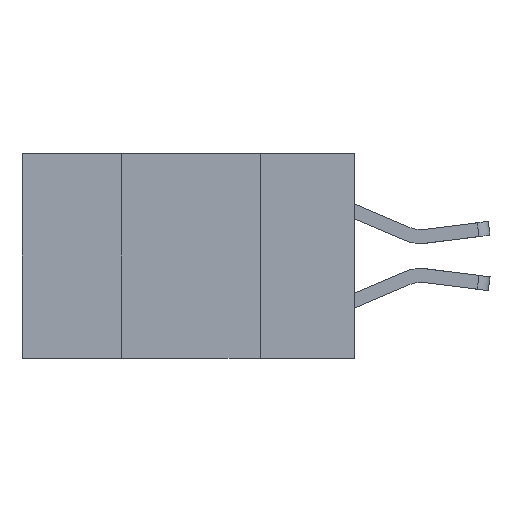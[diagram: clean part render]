
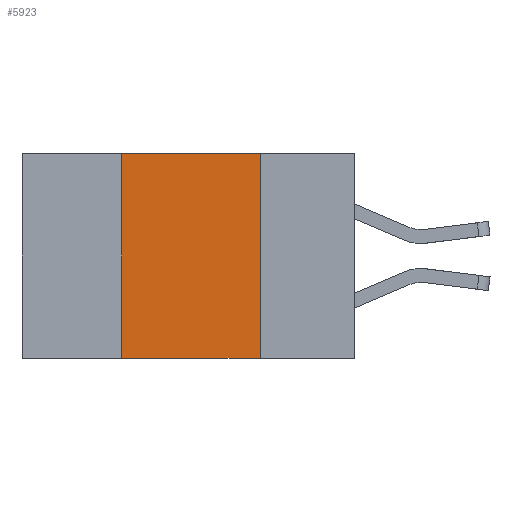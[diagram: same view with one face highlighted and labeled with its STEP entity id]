
A CAD part, left-side view. The second image highlights one B-rep face of the part: STEP entity #5923.
In plain terms, the highlighted planar face has unit normal (-1, 0, 0).
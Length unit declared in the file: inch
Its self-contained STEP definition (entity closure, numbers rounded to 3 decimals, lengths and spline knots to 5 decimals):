
#590 = CARTESIAN_POINT ( 'NONE',  ( 0., 0.17, 0. ) ) ;
#648 = VERTEX_POINT ( 'NONE', #7465 ) ;
#1519 = CARTESIAN_POINT ( 'NONE',  ( 0., 0.42, 0. ) ) ;
#1702 = EDGE_CURVE ( 'NONE', #5550, #648, #6798, .T. ) ;
#1976 = VECTOR ( 'NONE', #5303, 39.37008 ) ;
#2070 = EDGE_CURVE ( 'NONE', #648, #4972, #3769, .T. ) ;
#2094 = CARTESIAN_POINT ( 'NONE',  ( 0., 0.17, -0.37 ) ) ;
#2158 = CARTESIAN_POINT ( 'NONE',  ( 0., 0.6, -0.37 ) ) ;
#2169 = EDGE_CURVE ( 'NONE', #8180, #4972, #6313, .T. ) ;
#2476 = ORIENTED_EDGE ( 'NONE', *, *, #2169, .T. ) ;
#2839 = EDGE_LOOP ( 'NONE', ( #8367, #7723, #8049, #2476 ) ) ;
#3769 = LINE ( 'NONE', #590, #7121 ) ;
#3987 = CARTESIAN_POINT ( 'NONE',  ( 0., 0.6, 0. ) ) ;
#4972 = VERTEX_POINT ( 'NONE', #2094 ) ;
#4987 = CARTESIAN_POINT ( 'NONE',  ( 0., 0.42, 0. ) ) ;
#5043 = EDGE_CURVE ( 'NONE', #8180, #5550, #8377, .T. ) ;
#5303 = DIRECTION ( 'NONE',  ( 0., -1., 0. ) ) ;
#5388 = AXIS2_PLACEMENT_3D ( 'NONE', #9288, #5674, #9477 ) ;
#5518 = VECTOR ( 'NONE', #6897, 39.37008 ) ;
#5550 = VERTEX_POINT ( 'NONE', #4987 ) ;
#5674 = DIRECTION ( 'NONE',  ( 1., 0., 0. ) ) ;
#5704 = CARTESIAN_POINT ( 'NONE',  ( 0., 0.42, -0.37 ) ) ;
#5923 = ADVANCED_FACE ( 'NONE', ( #7161 ), #6278, .F. ) ;
#6258 = DIRECTION ( 'NONE',  ( 0., -1., 0. ) ) ;
#6278 = PLANE ( 'NONE',  #5388 ) ;
#6313 = LINE ( 'NONE', #2158, #1976 ) ;
#6798 = LINE ( 'NONE', #3987, #7028 ) ;
#6897 = DIRECTION ( 'NONE',  ( 0., 0., 1. ) ) ;
#7028 = VECTOR ( 'NONE', #6258, 39.37008 ) ;
#7121 = VECTOR ( 'NONE', #8847, 39.37008 ) ;
#7161 = FACE_OUTER_BOUND ( 'NONE', #2839, .T. ) ;
#7465 = CARTESIAN_POINT ( 'NONE',  ( 0., 0.17, 0. ) ) ;
#7723 = ORIENTED_EDGE ( 'NONE', *, *, #1702, .F. ) ;
#8049 = ORIENTED_EDGE ( 'NONE', *, *, #5043, .F. ) ;
#8180 = VERTEX_POINT ( 'NONE', #5704 ) ;
#8367 = ORIENTED_EDGE ( 'NONE', *, *, #2070, .F. ) ;
#8377 = LINE ( 'NONE', #1519, #5518 ) ;
#8847 = DIRECTION ( 'NONE',  ( 0., 0., -1. ) ) ;
#9288 = CARTESIAN_POINT ( 'NONE',  ( 0., 0.6, 0. ) ) ;
#9477 = DIRECTION ( 'NONE',  ( 0., 0., -1. ) ) ;
